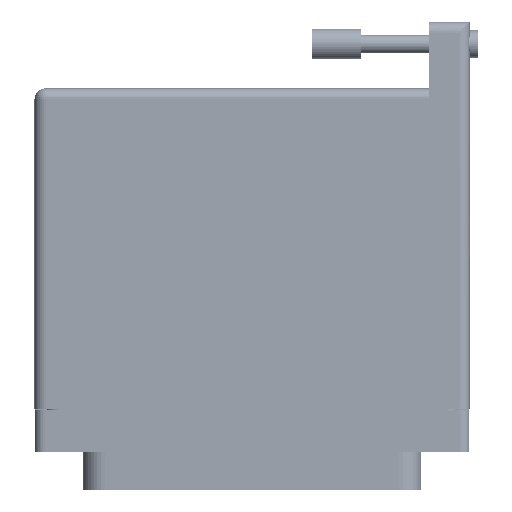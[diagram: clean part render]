
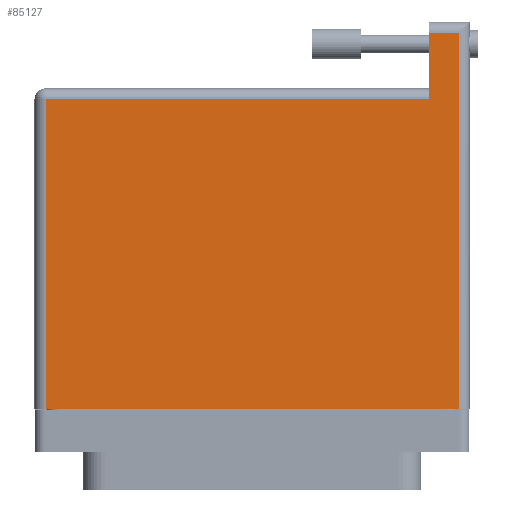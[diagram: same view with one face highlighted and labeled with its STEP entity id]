
A CAD part, front view. The second image highlights one B-rep face of the part: STEP entity #85127.
In plain terms, the highlighted face is planar.
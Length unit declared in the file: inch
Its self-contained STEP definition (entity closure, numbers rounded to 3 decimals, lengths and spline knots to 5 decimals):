
#3465 = CARTESIAN_POINT ( 'NONE',  ( -1.3775, 1.93, 0.765 ) ) ;
#3867 = EDGE_CURVE ( 'NONE', #4533, #9535, #22101, .T. ) ;
#4533 = VERTEX_POINT ( 'NONE', #24380 ) ;
#6626 = ORIENTED_EDGE ( 'NONE', *, *, #24408, .T. ) ;
#9535 = VERTEX_POINT ( 'NONE', #78764 ) ;
#10866 = DIRECTION ( 'NONE',  ( -1., 0., 0. ) ) ;
#11006 = FACE_OUTER_BOUND ( 'NONE', #49359, .T. ) ;
#11037 = LINE ( 'NONE', #42117, #41253 ) ;
#14687 = VERTEX_POINT ( 'NONE', #44137 ) ;
#18051 = DIRECTION ( 'NONE',  ( -1., 0., 0. ) ) ;
#22101 = LINE ( 'NONE', #38690, #90485 ) ;
#23016 = VERTEX_POINT ( 'NONE', #76026 ) ;
#24380 = CARTESIAN_POINT ( 'NONE',  ( 1.3075, 2.28, 0.765 ) ) ;
#24408 = EDGE_CURVE ( 'NONE', #9535, #89717, #81408, .T. ) ;
#24552 = ORIENTED_EDGE ( 'NONE', *, *, #52520, .T. ) ;
#27332 = VECTOR ( 'NONE', #52114, 39.37008 ) ;
#30557 = VERTEX_POINT ( 'NONE', #84672 ) ;
#32673 = CARTESIAN_POINT ( 'NONE',  ( 1.1215, 1.86, 0.765 ) ) ;
#32904 = PLANE ( 'NONE',  #69999 ) ;
#33155 = LINE ( 'NONE', #80432, #80258 ) ;
#36245 = LINE ( 'NONE', #45552, #27332 ) ;
#38690 = CARTESIAN_POINT ( 'NONE',  ( -1.3775, 2.28, 0.765 ) ) ;
#38826 = DIRECTION ( 'NONE',  ( 0., 0., -1. ) ) ;
#39069 = LINE ( 'NONE', #39557, #91833 ) ;
#39557 = CARTESIAN_POINT ( 'NONE',  ( -1.3775, 1.86, 0.765 ) ) ;
#41253 = VECTOR ( 'NONE', #55621, 39.37008 ) ;
#42117 = CARTESIAN_POINT ( 'NONE',  ( 1.3075, 2.35, 0.765 ) ) ;
#44137 = CARTESIAN_POINT ( 'NONE',  ( -1.3075, -0.1, 0.765 ) ) ;
#44305 = CARTESIAN_POINT ( 'NONE',  ( 1.1215, 2.35, 0.765 ) ) ;
#45552 = CARTESIAN_POINT ( 'NONE',  ( -1.3775, -0.1, 0.765 ) ) ;
#49359 = EDGE_LOOP ( 'NONE', ( #6626, #71463, #87463, #24552, #81167, #70888 ) ) ;
#50566 = EDGE_CURVE ( 'NONE', #89717, #30557, #39069, .T. ) ;
#52114 = DIRECTION ( 'NONE',  ( 1., 0., 0. ) ) ;
#52520 = EDGE_CURVE ( 'NONE', #14687, #23016, #36245, .T. ) ;
#53556 = DIRECTION ( 'NONE',  ( -1., 0., 0. ) ) ;
#55621 = DIRECTION ( 'NONE',  ( 0., 1., 0. ) ) ;
#57442 = DIRECTION ( 'NONE',  ( 0., -1., 0. ) ) ;
#63421 = VECTOR ( 'NONE', #57442, 39.37008 ) ;
#67941 = EDGE_CURVE ( 'NONE', #30557, #14687, #33155, .T. ) ;
#69999 = AXIS2_PLACEMENT_3D ( 'NONE', #3465, #38826, #53556 ) ;
#70888 = ORIENTED_EDGE ( 'NONE', *, *, #3867, .T. ) ;
#71463 = ORIENTED_EDGE ( 'NONE', *, *, #50566, .T. ) ;
#72580 = DIRECTION ( 'NONE',  ( 0., -1., 0. ) ) ;
#76026 = CARTESIAN_POINT ( 'NONE',  ( 1.3075, -0.1, 0.765 ) ) ;
#78764 = CARTESIAN_POINT ( 'NONE',  ( 1.1215, 2.28, 0.765 ) ) ;
#80258 = VECTOR ( 'NONE', #72580, 39.37008 ) ;
#80432 = CARTESIAN_POINT ( 'NONE',  ( -1.3075, -0.1, 0.765 ) ) ;
#81167 = ORIENTED_EDGE ( 'NONE', *, *, #90567, .T. ) ;
#81408 = LINE ( 'NONE', #44305, #63421 ) ;
#84672 = CARTESIAN_POINT ( 'NONE',  ( -1.3075, 1.86, 0.765 ) ) ;
#85127 = ADVANCED_FACE ( 'NONE', ( #11006 ), #32904, .F. ) ;
#87463 = ORIENTED_EDGE ( 'NONE', *, *, #67941, .T. ) ;
#89717 = VERTEX_POINT ( 'NONE', #32673 ) ;
#90485 = VECTOR ( 'NONE', #10866, 39.37008 ) ;
#90567 = EDGE_CURVE ( 'NONE', #23016, #4533, #11037, .T. ) ;
#91833 = VECTOR ( 'NONE', #18051, 39.37008 ) ;
